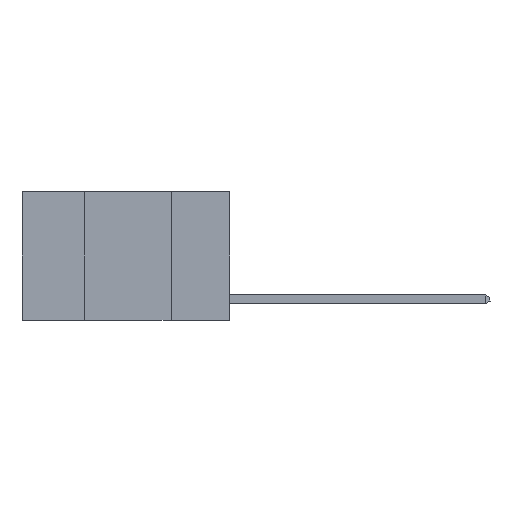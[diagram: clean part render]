
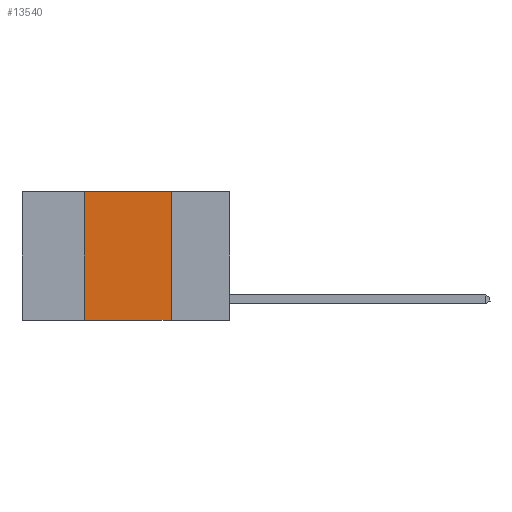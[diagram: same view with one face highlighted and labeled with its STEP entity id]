
A CAD part, left-side view. The second image highlights one B-rep face of the part: STEP entity #13540.
In plain terms, the highlighted planar face has unit normal (-1, 0, 0).
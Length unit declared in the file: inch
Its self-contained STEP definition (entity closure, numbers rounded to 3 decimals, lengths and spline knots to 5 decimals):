
#317 = FACE_OUTER_BOUND ( 'NONE', #2745, .T. ) ;
#1160 = CARTESIAN_POINT ( 'NONE',  ( 0., 0.6, 0. ) ) ;
#1989 = ORIENTED_EDGE ( 'NONE', *, *, #6634, .T. ) ;
#2745 = EDGE_LOOP ( 'NONE', ( #17682, #5059, #13821, #1989 ) ) ;
#2797 = DIRECTION ( 'NONE',  ( 0., -1., 0. ) ) ;
#3140 = DIRECTION ( 'NONE',  ( 0., 0., -1. ) ) ;
#3243 = CARTESIAN_POINT ( 'NONE',  ( 0., 0.17, 0. ) ) ;
#3695 = EDGE_CURVE ( 'NONE', #10787, #7106, #18675, .T. ) ;
#4163 = VECTOR ( 'NONE', #17623, 39.37008 ) ;
#4434 = CARTESIAN_POINT ( 'NONE',  ( 0., 0.42, 0. ) ) ;
#4440 = CARTESIAN_POINT ( 'NONE',  ( 0., 0.6, 0. ) ) ;
#4589 = DIRECTION ( 'NONE',  ( 0., -1., 0. ) ) ;
#5059 = ORIENTED_EDGE ( 'NONE', *, *, #17796, .F. ) ;
#5541 = VECTOR ( 'NONE', #3140, 39.37008 ) ;
#6125 = DIRECTION ( 'NONE',  ( 0., 0., -1. ) ) ;
#6634 = EDGE_CURVE ( 'NONE', #13166, #7106, #12897, .T. ) ;
#6807 = CARTESIAN_POINT ( 'NONE',  ( 0., 0.42, -0.37 ) ) ;
#7106 = VERTEX_POINT ( 'NONE', #21066 ) ;
#7378 = CARTESIAN_POINT ( 'NONE',  ( 0., 0.17, 0. ) ) ;
#9126 = LINE ( 'NONE', #4434, #4163 ) ;
#10546 = VECTOR ( 'NONE', #2797, 39.37008 ) ;
#10787 = VERTEX_POINT ( 'NONE', #7378 ) ;
#11476 = EDGE_CURVE ( 'NONE', #13166, #16952, #9126, .T. ) ;
#12084 = LINE ( 'NONE', #1160, #10546 ) ;
#12835 = CARTESIAN_POINT ( 'NONE',  ( 0., 0.6, -0.37 ) ) ;
#12897 = LINE ( 'NONE', #12835, #21064 ) ;
#13166 = VERTEX_POINT ( 'NONE', #6807 ) ;
#13540 = ADVANCED_FACE ( 'NONE', ( #317 ), #14330, .F. ) ;
#13719 = AXIS2_PLACEMENT_3D ( 'NONE', #4440, #15978, #6125 ) ;
#13821 = ORIENTED_EDGE ( 'NONE', *, *, #11476, .F. ) ;
#14330 = PLANE ( 'NONE',  #13719 ) ;
#15978 = DIRECTION ( 'NONE',  ( 1., 0., 0. ) ) ;
#16952 = VERTEX_POINT ( 'NONE', #18759 ) ;
#17623 = DIRECTION ( 'NONE',  ( 0., 0., 1. ) ) ;
#17682 = ORIENTED_EDGE ( 'NONE', *, *, #3695, .F. ) ;
#17796 = EDGE_CURVE ( 'NONE', #16952, #10787, #12084, .T. ) ;
#18675 = LINE ( 'NONE', #3243, #5541 ) ;
#18759 = CARTESIAN_POINT ( 'NONE',  ( 0., 0.42, 0. ) ) ;
#21064 = VECTOR ( 'NONE', #4589, 39.37008 ) ;
#21066 = CARTESIAN_POINT ( 'NONE',  ( 0., 0.17, -0.37 ) ) ;
